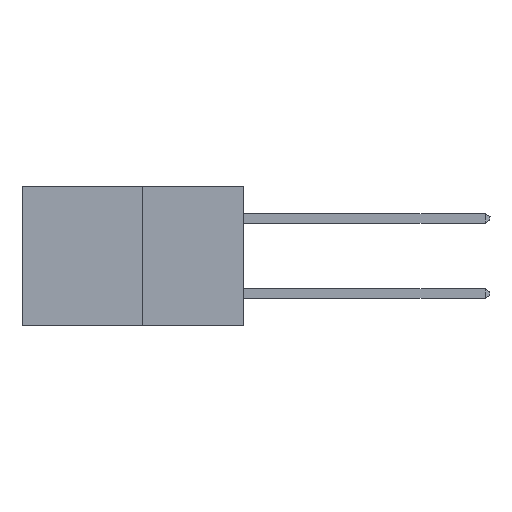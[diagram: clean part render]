
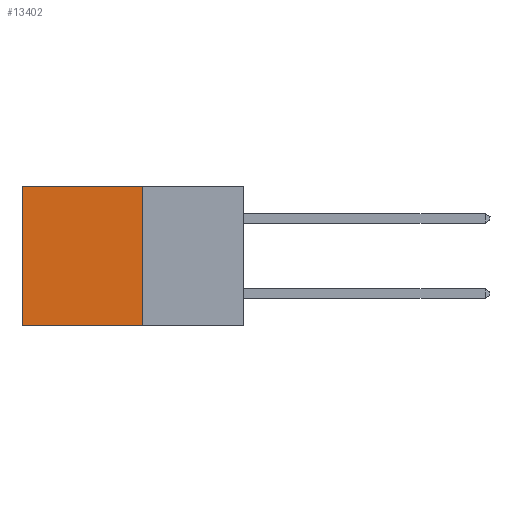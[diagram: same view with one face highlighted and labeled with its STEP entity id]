
A CAD part, left-side view. The second image highlights one B-rep face of the part: STEP entity #13402.
In plain terms, the highlighted planar face has unit normal (-1, 0, 0).
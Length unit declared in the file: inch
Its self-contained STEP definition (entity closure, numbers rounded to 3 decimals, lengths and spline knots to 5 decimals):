
#4 = VERTEX_POINT ( 'NONE', #11733 ) ;
#485 = CARTESIAN_POINT ( 'NONE',  ( 0.277, 0.27, -0.37 ) ) ;
#593 = VECTOR ( 'NONE', #1359, 39.37008 ) ;
#795 = CARTESIAN_POINT ( 'NONE',  ( 0.277, 0.27, -0.37 ) ) ;
#872 = VERTEX_POINT ( 'NONE', #4354 ) ;
#1359 = DIRECTION ( 'NONE',  ( 0., 0., -1. ) ) ;
#1481 = CARTESIAN_POINT ( 'NONE',  ( 0.277, 0.59, -0.37 ) ) ;
#1573 = CARTESIAN_POINT ( 'NONE',  ( 0.277, 0.59, -0.37 ) ) ;
#1913 = PLANE ( 'NONE',  #11118 ) ;
#1957 = DIRECTION ( 'NONE',  ( 0., 0., -1. ) ) ;
#2716 = VERTEX_POINT ( 'NONE', #1481 ) ;
#3027 = CARTESIAN_POINT ( 'NONE',  ( 0.277, 0.27, 0. ) ) ;
#3104 = DIRECTION ( 'NONE',  ( 1., 0., 0. ) ) ;
#3665 = ORIENTED_EDGE ( 'NONE', *, *, #11580, .T. ) ;
#3964 = VECTOR ( 'NONE', #1957, 39.37008 ) ;
#4170 = EDGE_CURVE ( 'NONE', #7855, #4, #12271, .T. ) ;
#4200 = EDGE_CURVE ( 'NONE', #872, #2716, #7408, .T. ) ;
#4351 = LINE ( 'NONE', #3027, #6809 ) ;
#4354 = CARTESIAN_POINT ( 'NONE',  ( 0.277, 0.59, 0. ) ) ;
#5139 = ORIENTED_EDGE ( 'NONE', *, *, #5434, .F. ) ;
#5434 = EDGE_CURVE ( 'NONE', #4, #2716, #9019, .T. ) ;
#5560 = EDGE_LOOP ( 'NONE', ( #9631, #5139, #9118, #3665 ) ) ;
#5621 = FACE_OUTER_BOUND ( 'NONE', #5560, .T. ) ;
#6273 = CARTESIAN_POINT ( 'NONE',  ( 0.277, 0.27, 0. ) ) ;
#6809 = VECTOR ( 'NONE', #11430, 39.37008 ) ;
#7408 = LINE ( 'NONE', #1573, #593 ) ;
#7855 = VERTEX_POINT ( 'NONE', #6273 ) ;
#9019 = LINE ( 'NONE', #11280, #13464 ) ;
#9118 = ORIENTED_EDGE ( 'NONE', *, *, #4170, .F. ) ;
#9631 = ORIENTED_EDGE ( 'NONE', *, *, #4200, .T. ) ;
#10477 = DIRECTION ( 'NONE',  ( 0., 0., -1. ) ) ;
#11118 = AXIS2_PLACEMENT_3D ( 'NONE', #795, #3104, #10477 ) ;
#11151 = DIRECTION ( 'NONE',  ( 0., 1., 0. ) ) ;
#11280 = CARTESIAN_POINT ( 'NONE',  ( 0.277, 0.27, -0.37 ) ) ;
#11430 = DIRECTION ( 'NONE',  ( 0., 1., 0. ) ) ;
#11580 = EDGE_CURVE ( 'NONE', #7855, #872, #4351, .T. ) ;
#11733 = CARTESIAN_POINT ( 'NONE',  ( 0.277, 0.27, -0.37 ) ) ;
#12271 = LINE ( 'NONE', #485, #3964 ) ;
#13402 = ADVANCED_FACE ( 'NONE', ( #5621 ), #1913, .F. ) ;
#13464 = VECTOR ( 'NONE', #11151, 39.37008 ) ;
